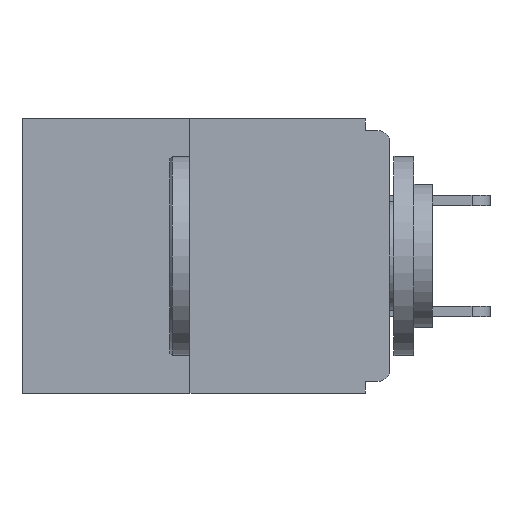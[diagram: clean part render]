
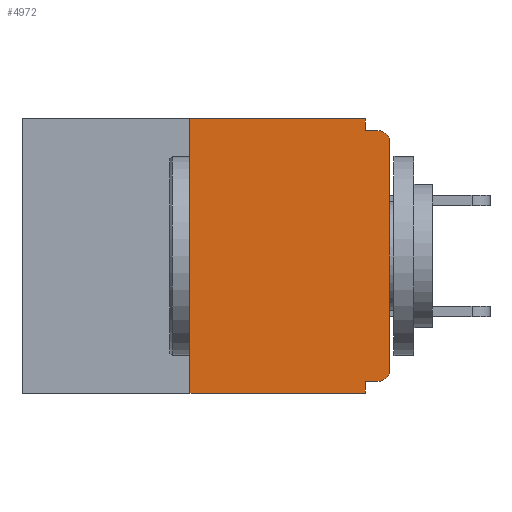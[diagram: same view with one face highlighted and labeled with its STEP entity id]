
A CAD part, left-side view. The second image highlights one B-rep face of the part: STEP entity #4972.
In plain terms, the highlighted planar face has unit normal (-1, 0, 0).
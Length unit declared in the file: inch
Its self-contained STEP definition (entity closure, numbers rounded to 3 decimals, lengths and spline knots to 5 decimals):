
#160 = ORIENTED_EDGE ( 'NONE', *, *, #7297, .F. ) ;
#362 = EDGE_CURVE ( 'NONE', #4074, #14073, #24189, .T. ) ;
#464 = CARTESIAN_POINT ( 'NONE',  ( 0., 0.015, -0.313 ) ) ;
#1086 = LINE ( 'NONE', #11760, #3243 ) ;
#2093 = CARTESIAN_POINT ( 'NONE',  ( 0., 0., -0.015 ) ) ;
#2144 = DIRECTION ( 'NONE',  ( -1., 0., 0. ) ) ;
#2733 = LINE ( 'NONE', #11119, #8180 ) ;
#2967 = VECTOR ( 'NONE', #5083, 39.37008 ) ;
#3243 = VECTOR ( 'NONE', #24608, 39.37008 ) ;
#3498 = EDGE_LOOP ( 'NONE', ( #24322, #24004, #24918, #10510, #160, #7541, #7671, #22376, #16935, #15661 ) ) ;
#3591 = EDGE_CURVE ( 'NONE', #16591, #7994, #1086, .T. ) ;
#3956 = DIRECTION ( 'NONE',  ( 0., 0., -1. ) ) ;
#4074 = VERTEX_POINT ( 'NONE', #16090 ) ;
#4353 = DIRECTION ( 'NONE',  ( -1., 0., 0. ) ) ;
#4599 = AXIS2_PLACEMENT_3D ( 'NONE', #19713, #2144, #17556 ) ;
#4638 = CARTESIAN_POINT ( 'NONE',  ( 0., 0.031, 0. ) ) ;
#4716 = VECTOR ( 'NONE', #22211, 39.37008 ) ;
#4972 = ADVANCED_FACE ( 'NONE', ( #7721 ), #5815, .F. ) ;
#5083 = DIRECTION ( 'NONE',  ( 0., 0., 1. ) ) ;
#5439 = DIRECTION ( 'NONE',  ( 0., 0., -1. ) ) ;
#5815 = PLANE ( 'NONE',  #13274 ) ;
#6207 = VERTEX_POINT ( 'NONE', #12348 ) ;
#6645 = DIRECTION ( 'NONE',  ( 0., -1., 0. ) ) ;
#6755 = CARTESIAN_POINT ( 'NONE',  ( 0., 0.25, 0. ) ) ;
#7297 = EDGE_CURVE ( 'NONE', #4074, #20948, #2733, .T. ) ;
#7541 = ORIENTED_EDGE ( 'NONE', *, *, #362, .T. ) ;
#7671 = ORIENTED_EDGE ( 'NONE', *, *, #22907, .T. ) ;
#7721 = FACE_OUTER_BOUND ( 'NONE', #3498, .T. ) ;
#7994 = VERTEX_POINT ( 'NONE', #15712 ) ;
#8180 = VECTOR ( 'NONE', #16951, 39.37008 ) ;
#8541 = CARTESIAN_POINT ( 'NONE',  ( 0., 0.46, 0. ) ) ;
#9745 = VECTOR ( 'NONE', #5439, 39.37008 ) ;
#9874 = CARTESIAN_POINT ( 'NONE',  ( 0., 0., -0.313 ) ) ;
#10510 = ORIENTED_EDGE ( 'NONE', *, *, #16021, .F. ) ;
#11119 = CARTESIAN_POINT ( 'NONE',  ( 0., 0., -0.328 ) ) ;
#11293 = LINE ( 'NONE', #2093, #13146 ) ;
#11491 = VECTOR ( 'NONE', #21613, 39.37008 ) ;
#11760 = CARTESIAN_POINT ( 'NONE',  ( 0., 0.46, -0.343 ) ) ;
#11790 = LINE ( 'NONE', #12843, #2967 ) ;
#11842 = CIRCLE ( 'NONE', #4599, 0.015 ) ;
#12206 = VERTEX_POINT ( 'NONE', #24597 ) ;
#12348 = CARTESIAN_POINT ( 'NONE',  ( 0., 0.015, -0.015 ) ) ;
#12843 = CARTESIAN_POINT ( 'NONE',  ( 0., 0., 0. ) ) ;
#13146 = VECTOR ( 'NONE', #6645, 39.37008 ) ;
#13241 = CARTESIAN_POINT ( 'NONE',  ( 0., 0., -0.03 ) ) ;
#13274 = AXIS2_PLACEMENT_3D ( 'NONE', #23356, #19481, #3956 ) ;
#13558 = VECTOR ( 'NONE', #14677, 39.37008 ) ;
#13802 = CARTESIAN_POINT ( 'NONE',  ( 0., 0.031, -0.343 ) ) ;
#14073 = VERTEX_POINT ( 'NONE', #9874 ) ;
#14285 = LINE ( 'NONE', #23319, #9745 ) ;
#14286 = EDGE_CURVE ( 'NONE', #16591, #18055, #25214, .T. ) ;
#14420 = VERTEX_POINT ( 'NONE', #13241 ) ;
#14677 = DIRECTION ( 'NONE',  ( 0., 0., 1. ) ) ;
#15319 = AXIS2_PLACEMENT_3D ( 'NONE', #464, #4353, #20475 ) ;
#15661 = ORIENTED_EDGE ( 'NONE', *, *, #21340, .F. ) ;
#15712 = CARTESIAN_POINT ( 'NONE',  ( 0., 0.031, -0.343 ) ) ;
#16021 = EDGE_CURVE ( 'NONE', #20948, #7994, #17317, .T. ) ;
#16090 = CARTESIAN_POINT ( 'NONE',  ( 0., 0.015, -0.328 ) ) ;
#16591 = VERTEX_POINT ( 'NONE', #22295 ) ;
#16935 = ORIENTED_EDGE ( 'NONE', *, *, #19836, .F. ) ;
#16951 = DIRECTION ( 'NONE',  ( 0., 1., 0. ) ) ;
#17317 = LINE ( 'NONE', #13802, #11491 ) ;
#17556 = DIRECTION ( 'NONE',  ( 0., 0., -1. ) ) ;
#18055 = VERTEX_POINT ( 'NONE', #22169 ) ;
#18505 = VERTEX_POINT ( 'NONE', #4638 ) ;
#19481 = DIRECTION ( 'NONE',  ( 1., 0., 0. ) ) ;
#19713 = CARTESIAN_POINT ( 'NONE',  ( 0., 0.015, -0.03 ) ) ;
#19836 = EDGE_CURVE ( 'NONE', #12206, #6207, #11293, .T. ) ;
#20475 = DIRECTION ( 'NONE',  ( 0., 0., -1. ) ) ;
#20948 = VERTEX_POINT ( 'NONE', #25062 ) ;
#21340 = EDGE_CURVE ( 'NONE', #18505, #12206, #14285, .T. ) ;
#21405 = EDGE_CURVE ( 'NONE', #14420, #6207, #11842, .T. ) ;
#21567 = LINE ( 'NONE', #8541, #4716 ) ;
#21613 = DIRECTION ( 'NONE',  ( 0., 0., -1. ) ) ;
#22169 = CARTESIAN_POINT ( 'NONE',  ( 0., 0.25, 0. ) ) ;
#22211 = DIRECTION ( 'NONE',  ( 0., -1., 0. ) ) ;
#22295 = CARTESIAN_POINT ( 'NONE',  ( 0., 0.25, -0.343 ) ) ;
#22376 = ORIENTED_EDGE ( 'NONE', *, *, #21405, .T. ) ;
#22907 = EDGE_CURVE ( 'NONE', #14073, #14420, #11790, .T. ) ;
#23319 = CARTESIAN_POINT ( 'NONE',  ( 0., 0.031, 0. ) ) ;
#23356 = CARTESIAN_POINT ( 'NONE',  ( 0., 0.46, 0. ) ) ;
#23871 = EDGE_CURVE ( 'NONE', #18055, #18505, #21567, .T. ) ;
#24004 = ORIENTED_EDGE ( 'NONE', *, *, #14286, .F. ) ;
#24189 = CIRCLE ( 'NONE', #15319, 0.015 ) ;
#24322 = ORIENTED_EDGE ( 'NONE', *, *, #23871, .F. ) ;
#24597 = CARTESIAN_POINT ( 'NONE',  ( 0., 0.031, -0.015 ) ) ;
#24608 = DIRECTION ( 'NONE',  ( 0., -1., 0. ) ) ;
#24918 = ORIENTED_EDGE ( 'NONE', *, *, #3591, .T. ) ;
#25062 = CARTESIAN_POINT ( 'NONE',  ( 0., 0.031, -0.328 ) ) ;
#25214 = LINE ( 'NONE', #6755, #13558 ) ;
